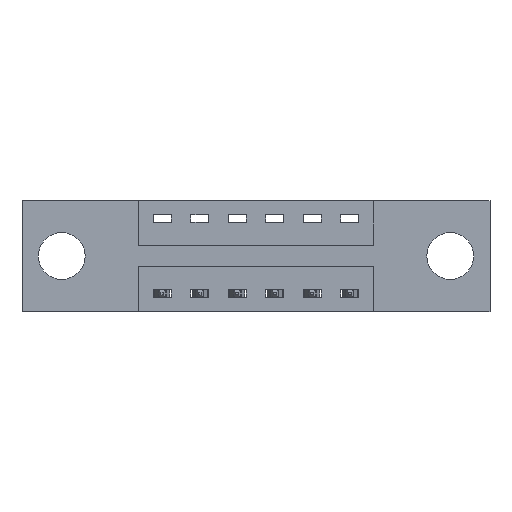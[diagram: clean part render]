
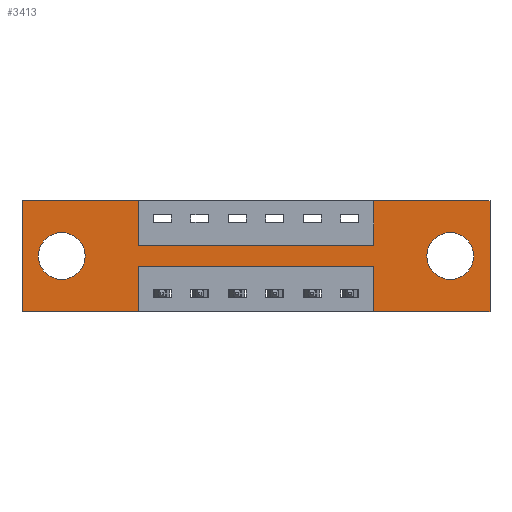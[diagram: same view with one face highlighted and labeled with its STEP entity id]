
A CAD part, front view. The second image highlights one B-rep face of the part: STEP entity #3413.
In plain terms, the highlighted planar face has unit normal (0, -1, 0).
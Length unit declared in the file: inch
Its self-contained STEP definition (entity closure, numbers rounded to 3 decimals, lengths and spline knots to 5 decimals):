
#113 = CARTESIAN_POINT ( 'NONE',  ( 1.1725, 0., 0. ) ) ;
#255 = DIRECTION ( 'NONE',  ( 0., 0., -1. ) ) ;
#281 = LINE ( 'NONE', #7596, #722 ) ;
#319 = ORIENTED_EDGE ( 'NONE', *, *, #6862, .F. ) ;
#371 = CARTESIAN_POINT ( 'NONE',  ( 0., 0., -0.37 ) ) ;
#425 = ORIENTED_EDGE ( 'NONE', *, *, #6682, .F. ) ;
#458 = LINE ( 'NONE', #4527, #5649 ) ;
#522 = VERTEX_POINT ( 'NONE', #4203 ) ;
#576 = ORIENTED_EDGE ( 'NONE', *, *, #4237, .F. ) ;
#634 = LINE ( 'NONE', #2154, #2415 ) ;
#636 = EDGE_LOOP ( 'NONE', ( #6293, #843 ) ) ;
#700 = EDGE_CURVE ( 'NONE', #6727, #522, #3059, .T. ) ;
#722 = VECTOR ( 'NONE', #8243, 39.37008 ) ;
#778 = AXIS2_PLACEMENT_3D ( 'NONE', #2655, #7293, #3423 ) ;
#804 = DIRECTION ( 'NONE',  ( 1., 0., 0. ) ) ;
#827 = ORIENTED_EDGE ( 'NONE', *, *, #700, .F. ) ;
#842 = DIRECTION ( 'NONE',  ( 0., 0., 1. ) ) ;
#843 = ORIENTED_EDGE ( 'NONE', *, *, #8566, .T. ) ;
#1135 = CARTESIAN_POINT ( 'NONE',  ( 0.3875, 0., -0.15 ) ) ;
#1210 = VECTOR ( 'NONE', #6515, 39.37008 ) ;
#1314 = CARTESIAN_POINT ( 'NONE',  ( 1.56, 0., -0.37 ) ) ;
#1318 = LINE ( 'NONE', #2347, #2476 ) ;
#1322 = CARTESIAN_POINT ( 'NONE',  ( 0.3875, 0., -0.37 ) ) ;
#1348 = VECTOR ( 'NONE', #7678, 39.37008 ) ;
#1407 = AXIS2_PLACEMENT_3D ( 'NONE', #5721, #1649, #6352 ) ;
#1408 = LINE ( 'NONE', #5860, #1210 ) ;
#1493 = CIRCLE ( 'NONE', #4650, 0.078 ) ;
#1534 = VERTEX_POINT ( 'NONE', #5645 ) ;
#1587 = ORIENTED_EDGE ( 'NONE', *, *, #8307, .F. ) ;
#1593 = CARTESIAN_POINT ( 'NONE',  ( 1.56, 0., 0. ) ) ;
#1609 = EDGE_LOOP ( 'NONE', ( #2003, #4272 ) ) ;
#1649 = DIRECTION ( 'NONE',  ( 0., -1., 0. ) ) ;
#1700 = ORIENTED_EDGE ( 'NONE', *, *, #6834, .F. ) ;
#1933 = DIRECTION ( 'NONE',  ( 0., 0., 1. ) ) ;
#1950 = VERTEX_POINT ( 'NONE', #4867 ) ;
#2003 = ORIENTED_EDGE ( 'NONE', *, *, #7329, .T. ) ;
#2056 = ORIENTED_EDGE ( 'NONE', *, *, #4442, .F. ) ;
#2105 = EDGE_CURVE ( 'NONE', #2336, #6023, #2690, .T. ) ;
#2108 = CIRCLE ( 'NONE', #778, 0.078 ) ;
#2154 = CARTESIAN_POINT ( 'NONE',  ( 1.1725, 0., 0. ) ) ;
#2335 = CARTESIAN_POINT ( 'NONE',  ( 0.3875, 0., -0.37 ) ) ;
#2336 = VERTEX_POINT ( 'NONE', #6117 ) ;
#2347 = CARTESIAN_POINT ( 'NONE',  ( 0.3875, 0., 0. ) ) ;
#2415 = VECTOR ( 'NONE', #842, 39.37008 ) ;
#2418 = EDGE_LOOP ( 'NONE', ( #5281, #1700, #3731, #319, #1587, #2907, #5505, #7862, #425, #576, #827, #2056 ) ) ;
#2423 = FACE_BOUND ( 'NONE', #636, .T. ) ;
#2463 = CARTESIAN_POINT ( 'NONE',  ( 0.3875, 0., -0.22 ) ) ;
#2476 = VECTOR ( 'NONE', #6369, 39.37008 ) ;
#2655 = CARTESIAN_POINT ( 'NONE',  ( 0.1325, 0., -0.185 ) ) ;
#2690 = CIRCLE ( 'NONE', #7855, 0.078 ) ;
#2907 = ORIENTED_EDGE ( 'NONE', *, *, #4310, .F. ) ;
#2985 = LINE ( 'NONE', #1135, #4819 ) ;
#3059 = LINE ( 'NONE', #6059, #8273 ) ;
#3299 = VECTOR ( 'NONE', #4574, 39.37008 ) ;
#3413 = ADVANCED_FACE ( 'NONE', ( #5995, #2423, #7505 ), #5072, .T. ) ;
#3423 = DIRECTION ( 'NONE',  ( 0., 0., 1. ) ) ;
#3489 = EDGE_CURVE ( 'NONE', #8233, #4108, #2985, .T. ) ;
#3633 = CARTESIAN_POINT ( 'NONE',  ( 0., 0., 0. ) ) ;
#3698 = CARTESIAN_POINT ( 'NONE',  ( 1.4275, 0., -0.185 ) ) ;
#3731 = ORIENTED_EDGE ( 'NONE', *, *, #4567, .F. ) ;
#3732 = EDGE_CURVE ( 'NONE', #4108, #7276, #634, .T. ) ;
#3779 = VERTEX_POINT ( 'NONE', #7544 ) ;
#3820 = DIRECTION ( 'NONE',  ( 0., 0., -1. ) ) ;
#4108 = VERTEX_POINT ( 'NONE', #6697 ) ;
#4203 = CARTESIAN_POINT ( 'NONE',  ( 0., 0., 0. ) ) ;
#4237 = EDGE_CURVE ( 'NONE', #522, #1534, #8581, .T. ) ;
#4259 = CARTESIAN_POINT ( 'NONE',  ( 0., 0., 0. ) ) ;
#4272 = ORIENTED_EDGE ( 'NONE', *, *, #8130, .T. ) ;
#4310 = EDGE_CURVE ( 'NONE', #7276, #4432, #4609, .T. ) ;
#4374 = DIRECTION ( 'NONE',  ( 0., 0., -1. ) ) ;
#4414 = VECTOR ( 'NONE', #3820, 39.37008 ) ;
#4422 = DIRECTION ( 'NONE',  ( 0., 1., 0. ) ) ;
#4432 = VERTEX_POINT ( 'NONE', #1593 ) ;
#4442 = EDGE_CURVE ( 'NONE', #5534, #6727, #281, .T. ) ;
#4495 = CARTESIAN_POINT ( 'NONE',  ( 0.1325, 0., -0.185 ) ) ;
#4527 = CARTESIAN_POINT ( 'NONE',  ( 1.56, 0., 0. ) ) ;
#4567 = EDGE_CURVE ( 'NONE', #8090, #1950, #6690, .T. ) ;
#4574 = DIRECTION ( 'NONE',  ( -1., 0., 0. ) ) ;
#4609 = LINE ( 'NONE', #3633, #7787 ) ;
#4650 = AXIS2_PLACEMENT_3D ( 'NONE', #8230, #4422, #255 ) ;
#4819 = VECTOR ( 'NONE', #5821, 39.37008 ) ;
#4867 = CARTESIAN_POINT ( 'NONE',  ( 1.1725, 0., -0.22 ) ) ;
#5066 = CARTESIAN_POINT ( 'NONE',  ( 0.3875, 0., -0.15 ) ) ;
#5072 = PLANE ( 'NONE',  #1407 ) ;
#5134 = EDGE_CURVE ( 'NONE', #3779, #5534, #6073, .T. ) ;
#5146 = DIRECTION ( 'NONE',  ( 0., 0., -1. ) ) ;
#5281 = ORIENTED_EDGE ( 'NONE', *, *, #5134, .F. ) ;
#5292 = CARTESIAN_POINT ( 'NONE',  ( 1.4275, 0., -0.107 ) ) ;
#5505 = ORIENTED_EDGE ( 'NONE', *, *, #3732, .F. ) ;
#5534 = VERTEX_POINT ( 'NONE', #1322 ) ;
#5645 = CARTESIAN_POINT ( 'NONE',  ( 0.3875, 0., 0. ) ) ;
#5649 = VECTOR ( 'NONE', #5146, 39.37008 ) ;
#5721 = CARTESIAN_POINT ( 'NONE',  ( 0., 0., -0.37 ) ) ;
#5821 = DIRECTION ( 'NONE',  ( 1., 0., 0. ) ) ;
#5860 = CARTESIAN_POINT ( 'NONE',  ( 0., 0., -0.37 ) ) ;
#5995 = FACE_BOUND ( 'NONE', #1609, .T. ) ;
#6005 = DIRECTION ( 'NONE',  ( 0., 1., 0. ) ) ;
#6023 = VERTEX_POINT ( 'NONE', #8358 ) ;
#6053 = AXIS2_PLACEMENT_3D ( 'NONE', #3698, #8174, #4374 ) ;
#6059 = CARTESIAN_POINT ( 'NONE',  ( 0., 0., 0. ) ) ;
#6073 = LINE ( 'NONE', #2335, #4414 ) ;
#6117 = CARTESIAN_POINT ( 'NONE',  ( 0.1325, 0., -0.107 ) ) ;
#6165 = VERTEX_POINT ( 'NONE', #5292 ) ;
#6230 = CARTESIAN_POINT ( 'NONE',  ( 1.1725, 0., -0.37 ) ) ;
#6293 = ORIENTED_EDGE ( 'NONE', *, *, #2105, .T. ) ;
#6313 = VERTEX_POINT ( 'NONE', #1314 ) ;
#6352 = DIRECTION ( 'NONE',  ( 0., 0., -1. ) ) ;
#6369 = DIRECTION ( 'NONE',  ( 0., 0., -1. ) ) ;
#6423 = CARTESIAN_POINT ( 'NONE',  ( 1.1725, 0., -0.37 ) ) ;
#6424 = VERTEX_POINT ( 'NONE', #7396 ) ;
#6515 = DIRECTION ( 'NONE',  ( -1., 0., 0. ) ) ;
#6682 = EDGE_CURVE ( 'NONE', #1534, #8233, #1318, .T. ) ;
#6690 = LINE ( 'NONE', #6423, #1348 ) ;
#6697 = CARTESIAN_POINT ( 'NONE',  ( 1.1725, 0., -0.15 ) ) ;
#6727 = VERTEX_POINT ( 'NONE', #371 ) ;
#6834 = EDGE_CURVE ( 'NONE', #1950, #3779, #8455, .T. ) ;
#6862 = EDGE_CURVE ( 'NONE', #6313, #8090, #1408, .T. ) ;
#6956 = CIRCLE ( 'NONE', #6053, 0.078 ) ;
#7276 = VERTEX_POINT ( 'NONE', #113 ) ;
#7293 = DIRECTION ( 'NONE',  ( 0., 1., 0. ) ) ;
#7329 = EDGE_CURVE ( 'NONE', #6165, #6424, #6956, .T. ) ;
#7396 = CARTESIAN_POINT ( 'NONE',  ( 1.4275, 0., -0.263 ) ) ;
#7485 = DIRECTION ( 'NONE',  ( 1., 0., 0. ) ) ;
#7505 = FACE_OUTER_BOUND ( 'NONE', #2418, .T. ) ;
#7544 = CARTESIAN_POINT ( 'NONE',  ( 0.3875, 0., -0.22 ) ) ;
#7554 = DIRECTION ( 'NONE',  ( 0., 0., 1. ) ) ;
#7596 = CARTESIAN_POINT ( 'NONE',  ( 0., 0., -0.37 ) ) ;
#7678 = DIRECTION ( 'NONE',  ( 0., 0., 1. ) ) ;
#7787 = VECTOR ( 'NONE', #7485, 39.37008 ) ;
#7855 = AXIS2_PLACEMENT_3D ( 'NONE', #4495, #6005, #7554 ) ;
#7862 = ORIENTED_EDGE ( 'NONE', *, *, #3489, .F. ) ;
#8090 = VERTEX_POINT ( 'NONE', #6230 ) ;
#8130 = EDGE_CURVE ( 'NONE', #6424, #6165, #1493, .T. ) ;
#8174 = DIRECTION ( 'NONE',  ( 0., 1., 0. ) ) ;
#8230 = CARTESIAN_POINT ( 'NONE',  ( 1.4275, 0., -0.185 ) ) ;
#8233 = VERTEX_POINT ( 'NONE', #5066 ) ;
#8243 = DIRECTION ( 'NONE',  ( -1., 0., 0. ) ) ;
#8273 = VECTOR ( 'NONE', #1933, 39.37008 ) ;
#8307 = EDGE_CURVE ( 'NONE', #4432, #6313, #458, .T. ) ;
#8358 = CARTESIAN_POINT ( 'NONE',  ( 0.1325, 0., -0.263 ) ) ;
#8390 = VECTOR ( 'NONE', #804, 39.37008 ) ;
#8455 = LINE ( 'NONE', #2463, #3299 ) ;
#8566 = EDGE_CURVE ( 'NONE', #6023, #2336, #2108, .T. ) ;
#8581 = LINE ( 'NONE', #4259, #8390 ) ;
